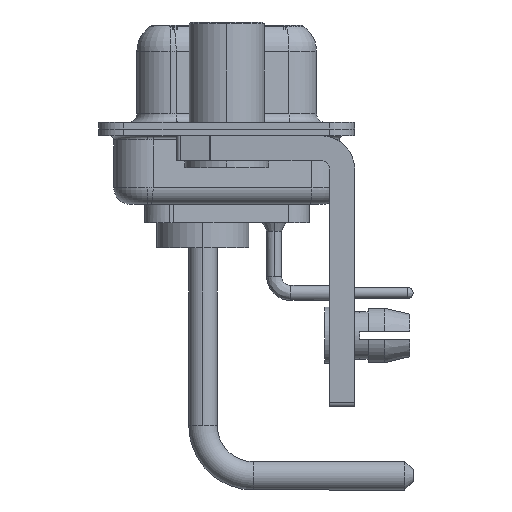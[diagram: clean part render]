
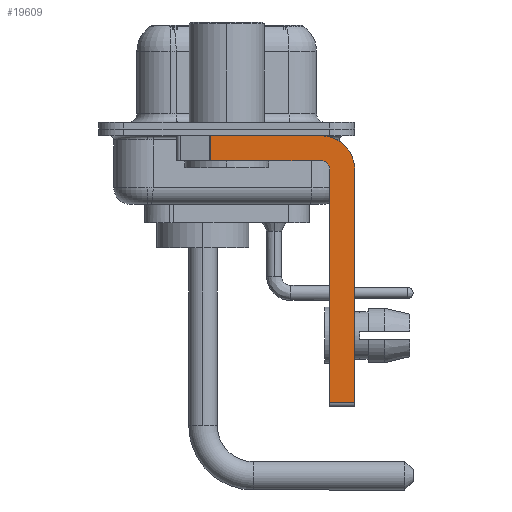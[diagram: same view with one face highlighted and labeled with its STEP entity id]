
A CAD part, left-side view. The second image highlights one B-rep face of the part: STEP entity #19609.
In plain terms, the highlighted planar face has unit normal (-1, 0, 0).
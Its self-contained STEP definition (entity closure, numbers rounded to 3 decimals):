
#216 = EDGE_CURVE ( 'NONE', #19987, #13354, #5484, .T. ) ;
#467 = VERTEX_POINT ( 'NONE', #7082 ) ;
#641 = DIRECTION ( 'NONE',  ( 0., 0., -1. ) ) ;
#1052 = EDGE_CURVE ( 'NONE', #7356, #13354, #16832, .T. ) ;
#1374 = CIRCLE ( 'NONE', #6989, 2. ) ;
#1977 = VECTOR ( 'NONE', #18827, 1000. ) ;
#2692 = ORIENTED_EDGE ( 'NONE', *, *, #8147, .F. ) ;
#2813 = EDGE_CURVE ( 'NONE', #19464, #6480, #17393, .T. ) ;
#2852 = CARTESIAN_POINT ( 'NONE',  ( -2.9, -6.15, -16.6 ) ) ;
#3988 = ORIENTED_EDGE ( 'NONE', *, *, #6854, .F. ) ;
#4762 = DIRECTION ( 'NONE',  ( -1., 0., 0. ) ) ;
#5036 = PLANE ( 'NONE',  #12172 ) ;
#5205 = CARTESIAN_POINT ( 'NONE',  ( -2.9, -7.65, -16.35 ) ) ;
#5484 = LINE ( 'NONE', #20751, #6699 ) ;
#5584 = DIRECTION ( 'NONE',  ( 0., -1., 0. ) ) ;
#5630 = CARTESIAN_POINT ( 'NONE',  ( -2.9, -6.15, -2.4 ) ) ;
#5923 = CARTESIAN_POINT ( 'NONE',  ( -2.9, -6.15, -16.35 ) ) ;
#6480 = VERTEX_POINT ( 'NONE', #5205 ) ;
#6647 = DIRECTION ( 'NONE',  ( 0., 0., 1. ) ) ;
#6699 = VECTOR ( 'NONE', #7613, 1000. ) ;
#6854 = EDGE_CURVE ( 'NONE', #467, #6480, #14094, .T. ) ;
#6989 = AXIS2_PLACEMENT_3D ( 'NONE', #14302, #8655, #19789 ) ;
#7082 = CARTESIAN_POINT ( 'NONE',  ( -2.9, -7.65, -2.4 ) ) ;
#7356 = VERTEX_POINT ( 'NONE', #21670 ) ;
#7613 = DIRECTION ( 'NONE',  ( 0., 1., 0. ) ) ;
#8064 = DIRECTION ( 'NONE',  ( 0., 0., -1. ) ) ;
#8068 = EDGE_LOOP ( 'NONE', ( #2692, #16621, #11804, #14247, #11962, #18211, #3988, #8727 ) ) ;
#8147 = EDGE_CURVE ( 'NONE', #7356, #17528, #15355, .T. ) ;
#8406 = CARTESIAN_POINT ( 'NONE',  ( -2.9, -5.65, -1.9 ) ) ;
#8448 = CARTESIAN_POINT ( 'NONE',  ( -2.9, -7.65, -2.4 ) ) ;
#8655 = DIRECTION ( 'NONE',  ( 1., 0., 0. ) ) ;
#8727 = ORIENTED_EDGE ( 'NONE', *, *, #19998, .F. ) ;
#10167 = DIRECTION ( 'NONE',  ( 1., 0., 0. ) ) ;
#10407 = EDGE_CURVE ( 'NONE', #10949, #19987, #11222, .T. ) ;
#10949 = VERTEX_POINT ( 'NONE', #5630 ) ;
#11222 = CIRCLE ( 'NONE', #22795, 0.5 ) ;
#11790 = VECTOR ( 'NONE', #8064, 1000. ) ;
#11804 = ORIENTED_EDGE ( 'NONE', *, *, #216, .F. ) ;
#11962 = ORIENTED_EDGE ( 'NONE', *, *, #23781, .F. ) ;
#12172 = AXIS2_PLACEMENT_3D ( 'NONE', #12676, #10167, #641 ) ;
#12676 = CARTESIAN_POINT ( 'NONE',  ( -2.9, -5.65, -2.4 ) ) ;
#13354 = VERTEX_POINT ( 'NONE', #16300 ) ;
#13969 = VECTOR ( 'NONE', #16268, 1000. ) ;
#14023 = LINE ( 'NONE', #2852, #13969 ) ;
#14094 = LINE ( 'NONE', #8448, #11790 ) ;
#14247 = ORIENTED_EDGE ( 'NONE', *, *, #10407, .F. ) ;
#14302 = CARTESIAN_POINT ( 'NONE',  ( -2.9, -5.65, -2.4 ) ) ;
#14574 = FACE_OUTER_BOUND ( 'NONE', #8068, .T. ) ;
#15355 = LINE ( 'NONE', #15470, #23168 ) ;
#15470 = CARTESIAN_POINT ( 'NONE',  ( -2.9, 3., -0.4 ) ) ;
#16268 = DIRECTION ( 'NONE',  ( 0., 0., 1. ) ) ;
#16300 = CARTESIAN_POINT ( 'NONE',  ( -2.9, 0.978, -1.9 ) ) ;
#16621 = ORIENTED_EDGE ( 'NONE', *, *, #1052, .T. ) ;
#16832 = LINE ( 'NONE', #22302, #1977 ) ;
#17393 = LINE ( 'NONE', #23128, #24725 ) ;
#17528 = VERTEX_POINT ( 'NONE', #20361 ) ;
#18211 = ORIENTED_EDGE ( 'NONE', *, *, #2813, .T. ) ;
#18827 = DIRECTION ( 'NONE',  ( 0., 0., -1. ) ) ;
#19464 = VERTEX_POINT ( 'NONE', #5923 ) ;
#19609 = ADVANCED_FACE ( 'NONE', ( #14574 ), #5036, .F. ) ;
#19789 = DIRECTION ( 'NONE',  ( 0., 0., -1. ) ) ;
#19987 = VERTEX_POINT ( 'NONE', #8406 ) ;
#19998 = EDGE_CURVE ( 'NONE', #17528, #467, #1374, .T. ) ;
#20361 = CARTESIAN_POINT ( 'NONE',  ( -2.9, -5.65, -0.4 ) ) ;
#20751 = CARTESIAN_POINT ( 'NONE',  ( -2.9, -5.65, -1.9 ) ) ;
#21375 = DIRECTION ( 'NONE',  ( 0., -1., 0. ) ) ;
#21670 = CARTESIAN_POINT ( 'NONE',  ( -2.9, 0.978, -0.4 ) ) ;
#22021 = CARTESIAN_POINT ( 'NONE',  ( -2.9, -5.65, -2.4 ) ) ;
#22302 = CARTESIAN_POINT ( 'NONE',  ( -2.9, 0.978, -1.9 ) ) ;
#22795 = AXIS2_PLACEMENT_3D ( 'NONE', #22021, #4762, #6647 ) ;
#23128 = CARTESIAN_POINT ( 'NONE',  ( -2.9, -5.65, -16.35 ) ) ;
#23168 = VECTOR ( 'NONE', #5584, 1000. ) ;
#23781 = EDGE_CURVE ( 'NONE', #19464, #10949, #14023, .T. ) ;
#24725 = VECTOR ( 'NONE', #21375, 1000. ) ;
